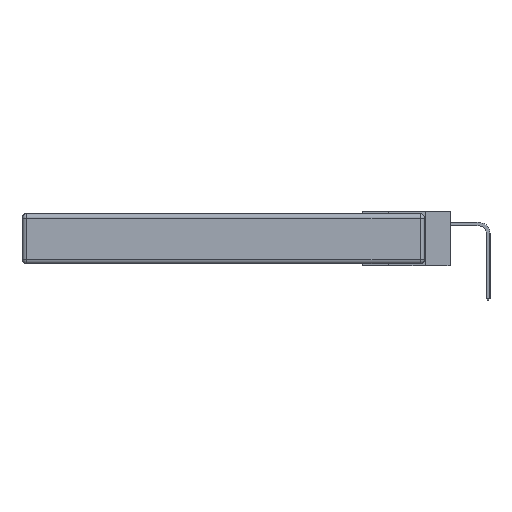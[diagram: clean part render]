
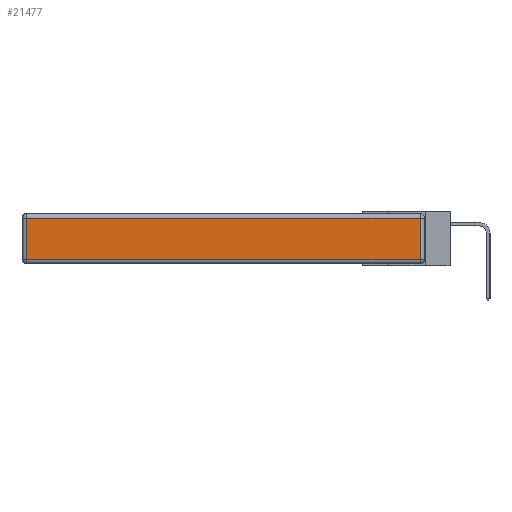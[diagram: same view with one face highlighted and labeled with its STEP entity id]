
A CAD part, left-side view. The second image highlights one B-rep face of the part: STEP entity #21477.
In plain terms, the highlighted planar face has unit normal (-1, 0, 0).
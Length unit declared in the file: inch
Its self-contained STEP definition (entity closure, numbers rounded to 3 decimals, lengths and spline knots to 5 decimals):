
#749 = LINE ( 'NONE', #23572, #6536 ) ;
#1666 = DIRECTION ( 'NONE',  ( 0., 0., 1. ) ) ;
#3929 = LINE ( 'NONE', #13688, #13812 ) ;
#4366 = CARTESIAN_POINT ( 'NONE',  ( 0., 2.72, -0.343 ) ) ;
#4402 = EDGE_CURVE ( 'NONE', #7375, #8046, #3929, .T. ) ;
#5072 = PLANE ( 'NONE',  #10687 ) ;
#6179 = VERTEX_POINT ( 'NONE', #21576 ) ;
#6523 = EDGE_CURVE ( 'NONE', #6179, #10267, #19110, .T. ) ;
#6536 = VECTOR ( 'NONE', #25856, 39.37008 ) ;
#7130 = DIRECTION ( 'NONE',  ( 0., 1., 0. ) ) ;
#7375 = VERTEX_POINT ( 'NONE', #25409 ) ;
#8046 = VERTEX_POINT ( 'NONE', #18924 ) ;
#8084 = ORIENTED_EDGE ( 'NONE', *, *, #6523, .T. ) ;
#10267 = VERTEX_POINT ( 'NONE', #16717 ) ;
#10687 = AXIS2_PLACEMENT_3D ( 'NONE', #18575, #21394, #1666 ) ;
#11301 = VECTOR ( 'NONE', #13122, 39.37008 ) ;
#12083 = ORIENTED_EDGE ( 'NONE', *, *, #4402, .T. ) ;
#12528 = EDGE_LOOP ( 'NONE', ( #8084, #22140, #12083, #19288 ) ) ;
#12837 = DIRECTION ( 'NONE',  ( 0., 0., -1. ) ) ;
#13122 = DIRECTION ( 'NONE',  ( 0., -1., 0. ) ) ;
#13688 = CARTESIAN_POINT ( 'NONE',  ( 0., 2.75, -0.03 ) ) ;
#13812 = VECTOR ( 'NONE', #7130, 39.37008 ) ;
#16717 = CARTESIAN_POINT ( 'NONE',  ( 0., 0.03, -0.313 ) ) ;
#16855 = FACE_OUTER_BOUND ( 'NONE', #12528, .T. ) ;
#18575 = CARTESIAN_POINT ( 'NONE',  ( 0., 0., -0.343 ) ) ;
#18924 = CARTESIAN_POINT ( 'NONE',  ( 0., 2.72, -0.03 ) ) ;
#19110 = LINE ( 'NONE', #21626, #11301 ) ;
#19288 = ORIENTED_EDGE ( 'NONE', *, *, #19446, .T. ) ;
#19446 = EDGE_CURVE ( 'NONE', #8046, #6179, #20435, .T. ) ;
#19982 = EDGE_CURVE ( 'NONE', #10267, #7375, #749, .T. ) ;
#20435 = LINE ( 'NONE', #4366, #27547 ) ;
#21394 = DIRECTION ( 'NONE',  ( -1., 0., 0. ) ) ;
#21477 = ADVANCED_FACE ( 'NONE', ( #16855 ), #5072, .T. ) ;
#21576 = CARTESIAN_POINT ( 'NONE',  ( 0., 2.72, -0.313 ) ) ;
#21626 = CARTESIAN_POINT ( 'NONE',  ( 0., 0., -0.313 ) ) ;
#22140 = ORIENTED_EDGE ( 'NONE', *, *, #19982, .T. ) ;
#23572 = CARTESIAN_POINT ( 'NONE',  ( 0., 0.03, -0.343 ) ) ;
#25409 = CARTESIAN_POINT ( 'NONE',  ( 0., 0.03, -0.03 ) ) ;
#25856 = DIRECTION ( 'NONE',  ( 0., 0., 1. ) ) ;
#27547 = VECTOR ( 'NONE', #12837, 39.37008 ) ;
